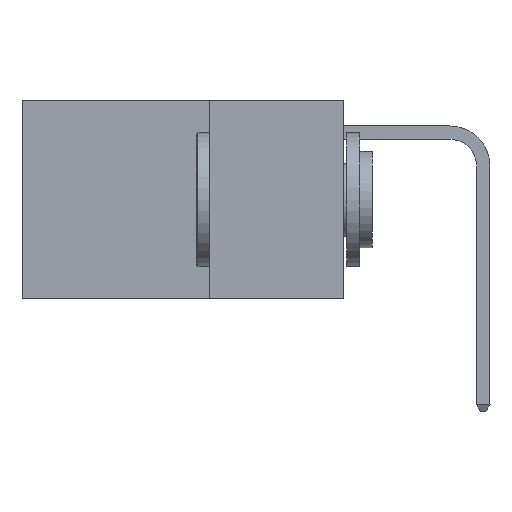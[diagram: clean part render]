
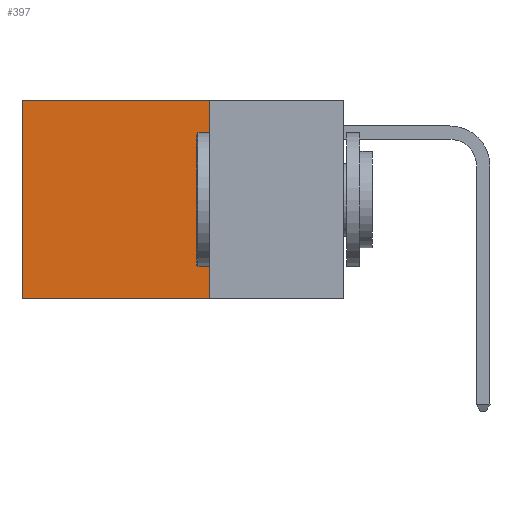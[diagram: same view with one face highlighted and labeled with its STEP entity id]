
A CAD part, left-side view. The second image highlights one B-rep face of the part: STEP entity #397.
In plain terms, the highlighted planar face has unit normal (-1, 0, 0).
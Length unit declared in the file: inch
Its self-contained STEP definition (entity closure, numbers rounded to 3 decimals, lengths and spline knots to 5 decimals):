
#397 = ADVANCED_FACE ( 'NONE', ( #5001 ), #5094, .F. ) ;
#682 = VECTOR ( 'NONE', #1441, 39.37008 ) ;
#695 = VERTEX_POINT ( 'NONE', #6295 ) ;
#851 = LINE ( 'NONE', #1477, #682 ) ;
#1299 = EDGE_CURVE ( 'NONE', #695, #4325, #3105, .T. ) ;
#1441 = DIRECTION ( 'NONE',  ( 0., 0., -1. ) ) ;
#1477 = CARTESIAN_POINT ( 'NONE',  ( 0.2625, 0.25, 0. ) ) ;
#1631 = AXIS2_PLACEMENT_3D ( 'NONE', #4942, #4990, #4858 ) ;
#2049 = ORIENTED_EDGE ( 'NONE', *, *, #4950, .T. ) ;
#2541 = CARTESIAN_POINT ( 'NONE',  ( 0.2625, 0.6, 0. ) ) ;
#2565 = DIRECTION ( 'NONE',  ( 0., 0., -1. ) ) ;
#3050 = VECTOR ( 'NONE', #7503, 39.37008 ) ;
#3105 = LINE ( 'NONE', #7476, #3050 ) ;
#3733 = EDGE_LOOP ( 'NONE', ( #2049, #5205, #5679, #5701 ) ) ;
#4059 = VERTEX_POINT ( 'NONE', #9157 ) ;
#4325 = VERTEX_POINT ( 'NONE', #7411 ) ;
#4457 = VECTOR ( 'NONE', #9419, 39.37008 ) ;
#4482 = LINE ( 'NONE', #9450, #4457 ) ;
#4858 = DIRECTION ( 'NONE',  ( 0., 0., -1. ) ) ;
#4942 = CARTESIAN_POINT ( 'NONE',  ( 0.2625, 0.25, 0. ) ) ;
#4950 = EDGE_CURVE ( 'NONE', #4059, #4325, #5406, .T. ) ;
#4990 = DIRECTION ( 'NONE',  ( 1., 0., 0. ) ) ;
#5001 = FACE_OUTER_BOUND ( 'NONE', #3733, .T. ) ;
#5094 = PLANE ( 'NONE',  #1631 ) ;
#5205 = ORIENTED_EDGE ( 'NONE', *, *, #1299, .F. ) ;
#5312 = VECTOR ( 'NONE', #2565, 39.37008 ) ;
#5406 = LINE ( 'NONE', #2541, #5312 ) ;
#5679 = ORIENTED_EDGE ( 'NONE', *, *, #10058, .F. ) ;
#5701 = ORIENTED_EDGE ( 'NONE', *, *, #8891, .T. ) ;
#6295 = CARTESIAN_POINT ( 'NONE',  ( 0.2625, 0.25, -0.37 ) ) ;
#7411 = CARTESIAN_POINT ( 'NONE',  ( 0.2625, 0.6, -0.37 ) ) ;
#7476 = CARTESIAN_POINT ( 'NONE',  ( 0.2625, 0.25, -0.37 ) ) ;
#7503 = DIRECTION ( 'NONE',  ( 0., 1., 0. ) ) ;
#8575 = CARTESIAN_POINT ( 'NONE',  ( 0.2625, 0.25, 0. ) ) ;
#8891 = EDGE_CURVE ( 'NONE', #8988, #4059, #4482, .T. ) ;
#8988 = VERTEX_POINT ( 'NONE', #8575 ) ;
#9157 = CARTESIAN_POINT ( 'NONE',  ( 0.2625, 0.6, 0. ) ) ;
#9419 = DIRECTION ( 'NONE',  ( 0., 1., 0. ) ) ;
#9450 = CARTESIAN_POINT ( 'NONE',  ( 0.2625, 0.25, 0. ) ) ;
#10058 = EDGE_CURVE ( 'NONE', #8988, #695, #851, .T. ) ;
